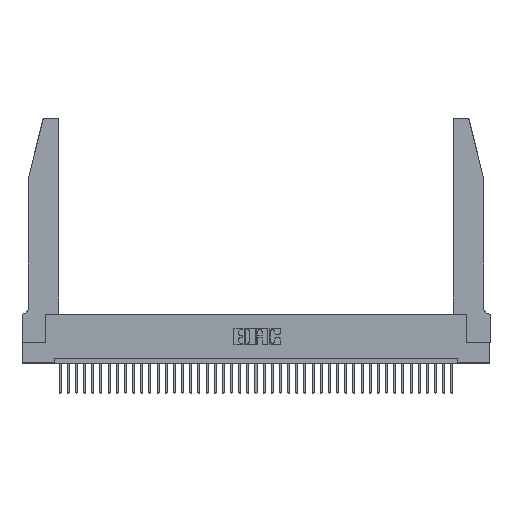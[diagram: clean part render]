
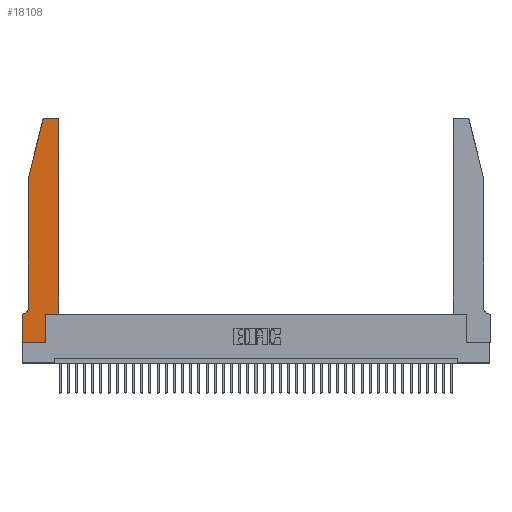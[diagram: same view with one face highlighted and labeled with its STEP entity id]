
A CAD part, top view. The second image highlights one B-rep face of the part: STEP entity #18108.
In plain terms, the highlighted planar face has unit normal (0, 0, 1).
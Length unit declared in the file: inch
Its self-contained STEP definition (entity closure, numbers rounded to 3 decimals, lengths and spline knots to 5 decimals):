
#140 = EDGE_CURVE ( 'NONE', #5157, #3550, #26238, .T. ) ;
#641 = CARTESIAN_POINT ( 'NONE',  ( 0.0755, 0.42, 0.37 ) ) ;
#676 = EDGE_CURVE ( 'NONE', #36017, #21688, #25286, .T. ) ;
#703 = EDGE_LOOP ( 'NONE', ( #38031, #12349, #38701, #23566, #2724, #22420, #34076, #10536, #20617, #39772, #989, #5214 ) ) ;
#974 = DIRECTION ( 'NONE',  ( -1., 0., 0. ) ) ;
#989 = ORIENTED_EDGE ( 'NONE', *, *, #7122, .T. ) ;
#1271 = LINE ( 'NONE', #27079, #20995 ) ;
#1288 = DIRECTION ( 'NONE',  ( 0., 0., 1. ) ) ;
#1474 = DIRECTION ( 'NONE',  ( -1., 0., 0. ) ) ;
#1713 = CARTESIAN_POINT ( 'NONE',  ( 0.2865, 0.35, 0.37 ) ) ;
#1888 = EDGE_CURVE ( 'NONE', #2126, #35504, #30130, .T. ) ;
#2045 = EDGE_CURVE ( 'NONE', #3550, #36017, #25181, .T. ) ;
#2126 = VERTEX_POINT ( 'NONE', #23799 ) ;
#2724 = ORIENTED_EDGE ( 'NONE', *, *, #12526, .T. ) ;
#3030 = AXIS2_PLACEMENT_3D ( 'NONE', #17179, #39116, #1474 ) ;
#3550 = VERTEX_POINT ( 'NONE', #29281 ) ;
#4295 = VERTEX_POINT ( 'NONE', #5098 ) ;
#4597 = CARTESIAN_POINT ( 'NONE',  ( 0.4505, 0.35, 0.37 ) ) ;
#4623 = EDGE_CURVE ( 'NONE', #35504, #4295, #11657, .T. ) ;
#5098 = CARTESIAN_POINT ( 'NONE',  ( 0.2865, 0., 0.37 ) ) ;
#5157 = VERTEX_POINT ( 'NONE', #14354 ) ;
#5214 = ORIENTED_EDGE ( 'NONE', *, *, #7003, .T. ) ;
#5298 = VERTEX_POINT ( 'NONE', #21316 ) ;
#7003 = EDGE_CURVE ( 'NONE', #17622, #5157, #18652, .T. ) ;
#7122 = EDGE_CURVE ( 'NONE', #33283, #17622, #30905, .T. ) ;
#7419 = CARTESIAN_POINT ( 'NONE',  ( 0., 0.35, 0.37 ) ) ;
#8559 = CARTESIAN_POINT ( 'NONE',  ( 0.0755, 2., 0.37 ) ) ;
#8578 = VECTOR ( 'NONE', #14890, 39.37008 ) ;
#9382 = LINE ( 'NONE', #1713, #28081 ) ;
#10405 = EDGE_CURVE ( 'NONE', #5298, #2126, #13320, .T. ) ;
#10536 = ORIENTED_EDGE ( 'NONE', *, *, #4623, .T. ) ;
#10818 = PLANE ( 'NONE',  #29870 ) ;
#11657 = LINE ( 'NONE', #34834, #34293 ) ;
#12349 = ORIENTED_EDGE ( 'NONE', *, *, #2045, .T. ) ;
#12526 = EDGE_CURVE ( 'NONE', #22154, #5298, #24809, .T. ) ;
#13320 = LINE ( 'NONE', #19544, #31118 ) ;
#13630 = CARTESIAN_POINT ( 'NONE',  ( 0.284, 2.72, 0.37 ) ) ;
#14070 = AXIS2_PLACEMENT_3D ( 'NONE', #13630, #35612, #29622 ) ;
#14354 = CARTESIAN_POINT ( 'NONE',  ( 0.4205, 2.75, 0.37 ) ) ;
#14890 = DIRECTION ( 'NONE',  ( 1., 0., 0. ) ) ;
#15783 = DIRECTION ( 'NONE',  ( 1., 0., 0. ) ) ;
#16125 = FACE_OUTER_BOUND ( 'NONE', #703, .T. ) ;
#16418 = EDGE_CURVE ( 'NONE', #21688, #22154, #1271, .T. ) ;
#16866 = AXIS2_PLACEMENT_3D ( 'NONE', #38923, #1288, #23320 ) ;
#17059 = CARTESIAN_POINT ( 'NONE',  ( 0., 0., 0.37 ) ) ;
#17179 = CARTESIAN_POINT ( 'NONE',  ( 0.0055, 0.42, 0.37 ) ) ;
#17418 = VECTOR ( 'NONE', #24027, 39.37008 ) ;
#17622 = VERTEX_POINT ( 'NONE', #35618 ) ;
#18108 = ADVANCED_FACE ( 'NONE', ( #16125 ), #10818, .T. ) ;
#18652 = CIRCLE ( 'NONE', #16866, 0.03 ) ;
#19544 = CARTESIAN_POINT ( 'NONE',  ( 0.0755, 0.35, 0.37 ) ) ;
#20424 = CARTESIAN_POINT ( 'NONE',  ( 0.2865, 0.35, 0.37 ) ) ;
#20474 = CARTESIAN_POINT ( 'NONE',  ( 0.0755, 2., 0.37 ) ) ;
#20617 = ORIENTED_EDGE ( 'NONE', *, *, #22512, .T. ) ;
#20750 = VECTOR ( 'NONE', #24055, 39.37008 ) ;
#20914 = EDGE_CURVE ( 'NONE', #24159, #33283, #38940, .T. ) ;
#20995 = VECTOR ( 'NONE', #35894, 39.37008 ) ;
#21230 = DIRECTION ( 'NONE',  ( -0.239, -0.971, 0. ) ) ;
#21285 = CARTESIAN_POINT ( 'NONE',  ( 0., 0., 0.37 ) ) ;
#21316 = CARTESIAN_POINT ( 'NONE',  ( 0.0055, 0.35, 0.37 ) ) ;
#21688 = VERTEX_POINT ( 'NONE', #8559 ) ;
#22154 = VERTEX_POINT ( 'NONE', #641 ) ;
#22420 = ORIENTED_EDGE ( 'NONE', *, *, #10405, .T. ) ;
#22512 = EDGE_CURVE ( 'NONE', #4295, #24159, #9382, .T. ) ;
#23320 = DIRECTION ( 'NONE',  ( 1., 0., 0. ) ) ;
#23566 = ORIENTED_EDGE ( 'NONE', *, *, #16418, .T. ) ;
#23740 = DIRECTION ( 'NONE',  ( 0., 1., 0. ) ) ;
#23799 = CARTESIAN_POINT ( 'NONE',  ( 0., 0.35, 0.37 ) ) ;
#24027 = DIRECTION ( 'NONE',  ( -1., 0., 0. ) ) ;
#24055 = DIRECTION ( 'NONE',  ( 0., -1., 0. ) ) ;
#24159 = VERTEX_POINT ( 'NONE', #20424 ) ;
#24809 = CIRCLE ( 'NONE', #3030, 0.07 ) ;
#25181 = CIRCLE ( 'NONE', #14070, 0.03 ) ;
#25286 = LINE ( 'NONE', #20474, #25776 ) ;
#25776 = VECTOR ( 'NONE', #21230, 39.37008 ) ;
#26238 = LINE ( 'NONE', #35343, #17418 ) ;
#27079 = CARTESIAN_POINT ( 'NONE',  ( 0.0755, 2., 0.37 ) ) ;
#28081 = VECTOR ( 'NONE', #33190, 39.37008 ) ;
#29281 = CARTESIAN_POINT ( 'NONE',  ( 0.284, 2.75, 0.37 ) ) ;
#29622 = DIRECTION ( 'NONE',  ( 1., 0., 0. ) ) ;
#29870 = AXIS2_PLACEMENT_3D ( 'NONE', #7419, #35668, #38965 ) ;
#30130 = LINE ( 'NONE', #21285, #20750 ) ;
#30469 = CARTESIAN_POINT ( 'NONE',  ( 0.4505, 0.35, 0.37 ) ) ;
#30905 = LINE ( 'NONE', #4597, #31838 ) ;
#31118 = VECTOR ( 'NONE', #974, 39.37008 ) ;
#31838 = VECTOR ( 'NONE', #23740, 39.37008 ) ;
#32649 = CARTESIAN_POINT ( 'NONE',  ( 0.4505, 0.35, 0.37 ) ) ;
#33190 = DIRECTION ( 'NONE',  ( 0., 1., 0. ) ) ;
#33283 = VERTEX_POINT ( 'NONE', #30469 ) ;
#34076 = ORIENTED_EDGE ( 'NONE', *, *, #1888, .T. ) ;
#34293 = VECTOR ( 'NONE', #15783, 39.37008 ) ;
#34834 = CARTESIAN_POINT ( 'NONE',  ( 0., 0., 0.37 ) ) ;
#35343 = CARTESIAN_POINT ( 'NONE',  ( 0.2605, 2.75, 0.37 ) ) ;
#35504 = VERTEX_POINT ( 'NONE', #17059 ) ;
#35612 = DIRECTION ( 'NONE',  ( 0., 0., 1. ) ) ;
#35618 = CARTESIAN_POINT ( 'NONE',  ( 0.4505, 2.72, 0.37 ) ) ;
#35668 = DIRECTION ( 'NONE',  ( 0., 0., 1. ) ) ;
#35894 = DIRECTION ( 'NONE',  ( 0., -1., 0. ) ) ;
#36017 = VERTEX_POINT ( 'NONE', #38530 ) ;
#38031 = ORIENTED_EDGE ( 'NONE', *, *, #140, .T. ) ;
#38530 = CARTESIAN_POINT ( 'NONE',  ( 0.25487, 2.72718, 0.37 ) ) ;
#38701 = ORIENTED_EDGE ( 'NONE', *, *, #676, .T. ) ;
#38923 = CARTESIAN_POINT ( 'NONE',  ( 0.4205, 2.72, 0.37 ) ) ;
#38940 = LINE ( 'NONE', #32649, #8578 ) ;
#38965 = DIRECTION ( 'NONE',  ( 1., 0., 0. ) ) ;
#39116 = DIRECTION ( 'NONE',  ( 0., 0., -1. ) ) ;
#39772 = ORIENTED_EDGE ( 'NONE', *, *, #20914, .T. ) ;
